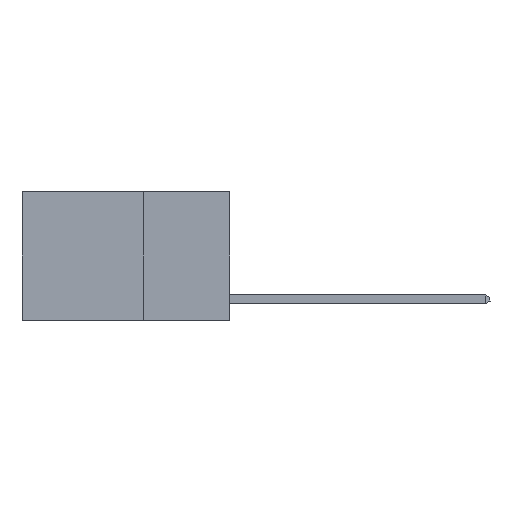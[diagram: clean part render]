
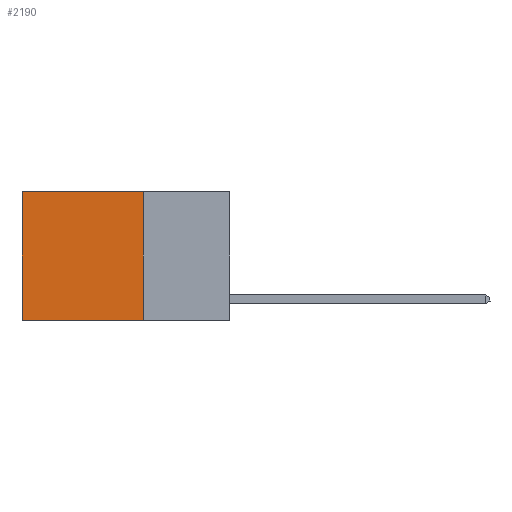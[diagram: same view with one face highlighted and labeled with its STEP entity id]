
A CAD part, left-side view. The second image highlights one B-rep face of the part: STEP entity #2190.
In plain terms, the highlighted planar face has unit normal (-1, 0, 0).
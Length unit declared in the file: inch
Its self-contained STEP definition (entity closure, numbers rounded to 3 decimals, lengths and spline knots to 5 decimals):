
#236 = VECTOR ( 'NONE', #10927, 39.37008 ) ;
#554 = LINE ( 'NONE', #9699, #3294 ) ;
#1120 = LINE ( 'NONE', #2807, #9965 ) ;
#1290 = CARTESIAN_POINT ( 'NONE',  ( 0.2625, 0.25, 0. ) ) ;
#2145 = VERTEX_POINT ( 'NONE', #7191 ) ;
#2190 = ADVANCED_FACE ( 'NONE', ( #10406 ), #3997, .F. ) ;
#2807 = CARTESIAN_POINT ( 'NONE',  ( 0.2625, 0.25, 0. ) ) ;
#3294 = VECTOR ( 'NONE', #6470, 39.37008 ) ;
#3647 = CARTESIAN_POINT ( 'NONE',  ( 0.2625, 0.6, 0. ) ) ;
#3997 = PLANE ( 'NONE',  #12378 ) ;
#4059 = EDGE_CURVE ( 'NONE', #2145, #13590, #14116, .T. ) ;
#5116 = CARTESIAN_POINT ( 'NONE',  ( 0.2625, 0.25, 0. ) ) ;
#5146 = ORIENTED_EDGE ( 'NONE', *, *, #7212, .T. ) ;
#5510 = CARTESIAN_POINT ( 'NONE',  ( 0.2625, 0.25, 0. ) ) ;
#5707 = EDGE_CURVE ( 'NONE', #7008, #12823, #9150, .T. ) ;
#6157 = ORIENTED_EDGE ( 'NONE', *, *, #7958, .F. ) ;
#6201 = DIRECTION ( 'NONE',  ( 0., 0., -1. ) ) ;
#6470 = DIRECTION ( 'NONE',  ( 0., 1., 0. ) ) ;
#6954 = CARTESIAN_POINT ( 'NONE',  ( 0.2625, 0.25, -0.37 ) ) ;
#7008 = VERTEX_POINT ( 'NONE', #1290 ) ;
#7191 = CARTESIAN_POINT ( 'NONE',  ( 0.2625, 0.6, 0. ) ) ;
#7212 = EDGE_CURVE ( 'NONE', #7008, #2145, #1120, .T. ) ;
#7958 = EDGE_CURVE ( 'NONE', #12823, #13590, #554, .T. ) ;
#8018 = EDGE_LOOP ( 'NONE', ( #9372, #6157, #12493, #5146 ) ) ;
#8865 = VECTOR ( 'NONE', #10173, 39.37008 ) ;
#9150 = LINE ( 'NONE', #5510, #236 ) ;
#9372 = ORIENTED_EDGE ( 'NONE', *, *, #4059, .T. ) ;
#9699 = CARTESIAN_POINT ( 'NONE',  ( 0.2625, 0.25, -0.37 ) ) ;
#9965 = VECTOR ( 'NONE', #11521, 39.37008 ) ;
#10173 = DIRECTION ( 'NONE',  ( 0., 0., -1. ) ) ;
#10406 = FACE_OUTER_BOUND ( 'NONE', #8018, .T. ) ;
#10927 = DIRECTION ( 'NONE',  ( 0., 0., -1. ) ) ;
#11521 = DIRECTION ( 'NONE',  ( 0., 1., 0. ) ) ;
#12378 = AXIS2_PLACEMENT_3D ( 'NONE', #5116, #12612, #6201 ) ;
#12493 = ORIENTED_EDGE ( 'NONE', *, *, #5707, .F. ) ;
#12612 = DIRECTION ( 'NONE',  ( 1., 0., 0. ) ) ;
#12823 = VERTEX_POINT ( 'NONE', #6954 ) ;
#13490 = CARTESIAN_POINT ( 'NONE',  ( 0.2625, 0.6, -0.37 ) ) ;
#13590 = VERTEX_POINT ( 'NONE', #13490 ) ;
#14116 = LINE ( 'NONE', #3647, #8865 ) ;
